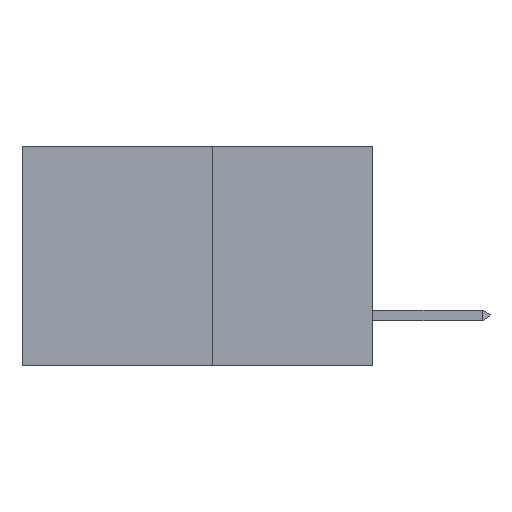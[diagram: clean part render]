
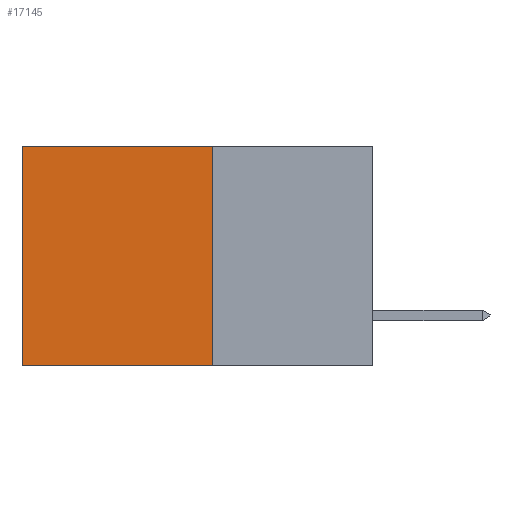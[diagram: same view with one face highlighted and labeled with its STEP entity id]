
A CAD part, left-side view. The second image highlights one B-rep face of the part: STEP entity #17145.
In plain terms, the highlighted planar face has unit normal (-1, 0, 0).
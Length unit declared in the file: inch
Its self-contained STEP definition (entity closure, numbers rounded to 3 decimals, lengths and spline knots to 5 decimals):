
#891 = LINE ( 'NONE', #6966, #12475 ) ;
#1191 = EDGE_CURVE ( 'NONE', #5140, #15974, #27718, .T. ) ;
#1828 = CARTESIAN_POINT ( 'NONE',  ( 0.277, 0.27, -0.37 ) ) ;
#1853 = VECTOR ( 'NONE', #14876, 39.37008 ) ;
#3343 = LINE ( 'NONE', #26476, #1853 ) ;
#3484 = CARTESIAN_POINT ( 'NONE',  ( 0.277, 0.59, -0.37 ) ) ;
#4524 = CARTESIAN_POINT ( 'NONE',  ( 0.277, 0.27, -0.37 ) ) ;
#5140 = VERTEX_POINT ( 'NONE', #18370 ) ;
#5800 = VERTEX_POINT ( 'NONE', #28653 ) ;
#6297 = PLANE ( 'NONE',  #23083 ) ;
#6368 = DIRECTION ( 'NONE',  ( 0., 1., 0. ) ) ;
#6564 = ORIENTED_EDGE ( 'NONE', *, *, #29343, .T. ) ;
#6966 = CARTESIAN_POINT ( 'NONE',  ( 0.277, 0.59, -0.37 ) ) ;
#8432 = ORIENTED_EDGE ( 'NONE', *, *, #12486, .T. ) ;
#8608 = DIRECTION ( 'NONE',  ( 0., 0., -1. ) ) ;
#9264 = DIRECTION ( 'NONE',  ( 0., 0., -1. ) ) ;
#10361 = VERTEX_POINT ( 'NONE', #3484 ) ;
#12475 = VECTOR ( 'NONE', #9264, 39.37008 ) ;
#12486 = EDGE_CURVE ( 'NONE', #5140, #5800, #23205, .T. ) ;
#14876 = DIRECTION ( 'NONE',  ( 0., 1., 0. ) ) ;
#15974 = VERTEX_POINT ( 'NONE', #1828 ) ;
#16421 = EDGE_LOOP ( 'NONE', ( #6564, #28179, #17659, #8432 ) ) ;
#17000 = VECTOR ( 'NONE', #6368, 39.37008 ) ;
#17145 = ADVANCED_FACE ( 'NONE', ( #22321 ), #6297, .F. ) ;
#17659 = ORIENTED_EDGE ( 'NONE', *, *, #1191, .F. ) ;
#17913 = CARTESIAN_POINT ( 'NONE',  ( 0.277, 0.27, -0.37 ) ) ;
#18370 = CARTESIAN_POINT ( 'NONE',  ( 0.277, 0.27, 0. ) ) ;
#20858 = DIRECTION ( 'NONE',  ( 0., 0., -1. ) ) ;
#21590 = VECTOR ( 'NONE', #20858, 39.37008 ) ;
#22321 = FACE_OUTER_BOUND ( 'NONE', #16421, .T. ) ;
#22575 = DIRECTION ( 'NONE',  ( 1., 0., 0. ) ) ;
#22652 = CARTESIAN_POINT ( 'NONE',  ( 0.277, 0.27, 0. ) ) ;
#23083 = AXIS2_PLACEMENT_3D ( 'NONE', #17913, #22575, #8608 ) ;
#23205 = LINE ( 'NONE', #22652, #17000 ) ;
#24891 = EDGE_CURVE ( 'NONE', #15974, #10361, #3343, .T. ) ;
#26476 = CARTESIAN_POINT ( 'NONE',  ( 0.277, 0.27, -0.37 ) ) ;
#27718 = LINE ( 'NONE', #4524, #21590 ) ;
#28179 = ORIENTED_EDGE ( 'NONE', *, *, #24891, .F. ) ;
#28653 = CARTESIAN_POINT ( 'NONE',  ( 0.277, 0.59, 0. ) ) ;
#29343 = EDGE_CURVE ( 'NONE', #5800, #10361, #891, .T. ) ;
